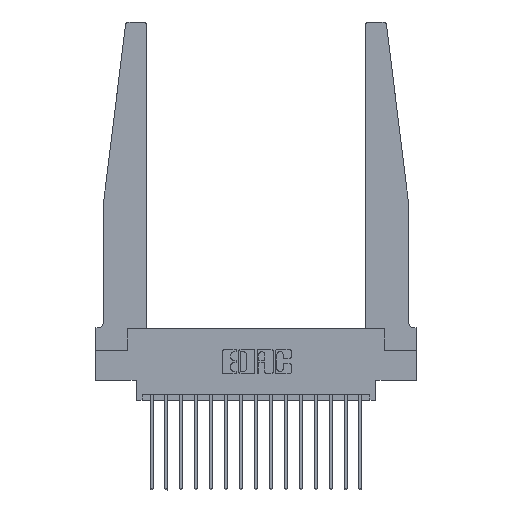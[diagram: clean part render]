
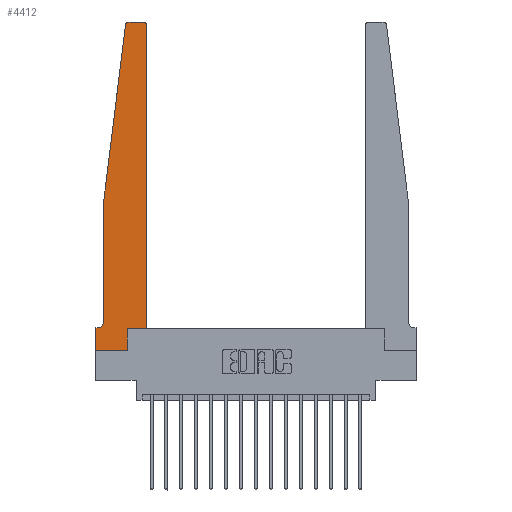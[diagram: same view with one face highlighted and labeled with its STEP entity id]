
A CAD part, top view. The second image highlights one B-rep face of the part: STEP entity #4412.
In plain terms, the highlighted planar face has unit normal (0, 0, 1).
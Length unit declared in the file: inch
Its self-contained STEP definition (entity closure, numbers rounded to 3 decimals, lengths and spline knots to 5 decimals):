
#121 = ORIENTED_EDGE ( 'NONE', *, *, #9849, .T. ) ;
#164 = DIRECTION ( 'NONE',  ( 1., 0., 0. ) ) ;
#223 = LINE ( 'NONE', #15361, #18182 ) ;
#229 = DIRECTION ( 'NONE',  ( 1., 0., 0. ) ) ;
#516 = LINE ( 'NONE', #5419, #961 ) ;
#643 = VECTOR ( 'NONE', #4997, 39.37008 ) ;
#768 = VERTEX_POINT ( 'NONE', #7733 ) ;
#961 = VECTOR ( 'NONE', #12491, 39.37008 ) ;
#1172 = VERTEX_POINT ( 'NONE', #8192 ) ;
#1193 = EDGE_CURVE ( 'NONE', #768, #3084, #7460, .T. ) ;
#1429 = EDGE_CURVE ( 'NONE', #5966, #18178, #14309, .T. ) ;
#2091 = VERTEX_POINT ( 'NONE', #11715 ) ;
#2338 = EDGE_CURVE ( 'NONE', #12616, #2091, #516, .T. ) ;
#2660 = ORIENTED_EDGE ( 'NONE', *, *, #11470, .T. ) ;
#2821 = ORIENTED_EDGE ( 'NONE', *, *, #5171, .T. ) ;
#2945 = PLANE ( 'NONE',  #18149 ) ;
#2963 = CARTESIAN_POINT ( 'NONE',  ( 0., 0., 0.37 ) ) ;
#3084 = VERTEX_POINT ( 'NONE', #2963 ) ;
#3543 = ORIENTED_EDGE ( 'NONE', *, *, #1429, .T. ) ;
#3628 = CARTESIAN_POINT ( 'NONE',  ( 0.425, 0.18, 0.37 ) ) ;
#4214 = EDGE_CURVE ( 'NONE', #9185, #15497, #4988, .T. ) ;
#4399 = AXIS2_PLACEMENT_3D ( 'NONE', #17159, #8705, #164 ) ;
#4412 = ADVANCED_FACE ( 'NONE', ( #16954 ), #2945, .T. ) ;
#4439 = CARTESIAN_POINT ( 'NONE',  ( 0., 0.1875, 0.37 ) ) ;
#4670 = DIRECTION ( 'NONE',  ( 1., 0., 0. ) ) ;
#4988 = LINE ( 'NONE', #9378, #15846 ) ;
#4997 = DIRECTION ( 'NONE',  ( -1., 0., 0. ) ) ;
#5057 = VERTEX_POINT ( 'NONE', #14268 ) ;
#5171 = EDGE_CURVE ( 'NONE', #3084, #9029, #9197, .T. ) ;
#5419 = CARTESIAN_POINT ( 'NONE',  ( 0.065, 1.25, 0.37 ) ) ;
#5646 = EDGE_CURVE ( 'NONE', #15497, #1172, #17139, .T. ) ;
#5870 = DIRECTION ( 'NONE',  ( 1., 0., 0. ) ) ;
#5888 = CARTESIAN_POINT ( 'NONE',  ( 0.425, 0.18, 0.37 ) ) ;
#5966 = VERTEX_POINT ( 'NONE', #6827 ) ;
#6375 = CARTESIAN_POINT ( 'NONE',  ( 0.065, 0.1875, 0.37 ) ) ;
#6827 = CARTESIAN_POINT ( 'NONE',  ( 0.2605, 0.18, 0.37 ) ) ;
#6844 = CARTESIAN_POINT ( 'NONE',  ( 0., 0., 0.37 ) ) ;
#7391 = CARTESIAN_POINT ( 'NONE',  ( 0.065, 1.25, 0.37 ) ) ;
#7449 = ORIENTED_EDGE ( 'NONE', *, *, #2338, .T. ) ;
#7460 = LINE ( 'NONE', #6844, #14083 ) ;
#7733 = CARTESIAN_POINT ( 'NONE',  ( 0., 0.1875, 0.37 ) ) ;
#7759 = DIRECTION ( 'NONE',  ( 0., 0., -1. ) ) ;
#7791 = EDGE_LOOP ( 'NONE', ( #11201, #15063, #15660, #7449, #16136, #2660, #10846, #2821, #9640, #3543, #15742, #121 ) ) ;
#7834 = AXIS2_PLACEMENT_3D ( 'NONE', #16225, #7759, #17645 ) ;
#7994 = DIRECTION ( 'NONE',  ( -1., 0., 0. ) ) ;
#8192 = CARTESIAN_POINT ( 'NONE',  ( 0.24675, 2.72367, 0.37 ) ) ;
#8348 = DIRECTION ( 'NONE',  ( 0., 0., 1. ) ) ;
#8705 = DIRECTION ( 'NONE',  ( 0., 0., 1. ) ) ;
#9029 = VERTEX_POINT ( 'NONE', #11405 ) ;
#9185 = VERTEX_POINT ( 'NONE', #10270 ) ;
#9197 = LINE ( 'NONE', #14562, #12951 ) ;
#9378 = CARTESIAN_POINT ( 'NONE',  ( 0.25, 2.75, 0.37 ) ) ;
#9390 = LINE ( 'NONE', #3628, #16900 ) ;
#9640 = ORIENTED_EDGE ( 'NONE', *, *, #11027, .T. ) ;
#9849 = EDGE_CURVE ( 'NONE', #15060, #9185, #13245, .T. ) ;
#9928 = CARTESIAN_POINT ( 'NONE',  ( 0.065, 1.25, 0.37 ) ) ;
#10068 = LINE ( 'NONE', #7391, #13785 ) ;
#10270 = CARTESIAN_POINT ( 'NONE',  ( 0.395, 2.75, 0.37 ) ) ;
#10390 = CIRCLE ( 'NONE', #7834, 0.05 ) ;
#10846 = ORIENTED_EDGE ( 'NONE', *, *, #1193, .T. ) ;
#11027 = EDGE_CURVE ( 'NONE', #9029, #5966, #223, .T. ) ;
#11198 = DIRECTION ( 'NONE',  ( 0., 1., 0. ) ) ;
#11201 = ORIENTED_EDGE ( 'NONE', *, *, #4214, .T. ) ;
#11405 = CARTESIAN_POINT ( 'NONE',  ( 0.2605, 0., 0.37 ) ) ;
#11470 = EDGE_CURVE ( 'NONE', #5057, #768, #15737, .T. ) ;
#11715 = CARTESIAN_POINT ( 'NONE',  ( 0.065, 0.2375, 0.37 ) ) ;
#12491 = DIRECTION ( 'NONE',  ( 0., -1., 0. ) ) ;
#12616 = VERTEX_POINT ( 'NONE', #9928 ) ;
#12951 = VECTOR ( 'NONE', #4670, 39.37008 ) ;
#13020 = DIRECTION ( 'NONE',  ( -0.122, -0.992, 0. ) ) ;
#13245 = CIRCLE ( 'NONE', #18094, 0.03 ) ;
#13548 = DIRECTION ( 'NONE',  ( 0., 1., 0. ) ) ;
#13785 = VECTOR ( 'NONE', #13020, 39.37008 ) ;
#13861 = DIRECTION ( 'NONE',  ( 0., -1., 0. ) ) ;
#14070 = EDGE_CURVE ( 'NONE', #2091, #5057, #10390, .T. ) ;
#14083 = VECTOR ( 'NONE', #13861, 39.37008 ) ;
#14268 = CARTESIAN_POINT ( 'NONE',  ( 0.015, 0.1875, 0.37 ) ) ;
#14309 = LINE ( 'NONE', #5888, #15180 ) ;
#14352 = DIRECTION ( 'NONE',  ( 0., 0., 1. ) ) ;
#14562 = CARTESIAN_POINT ( 'NONE',  ( 0., 0., 0.37 ) ) ;
#15060 = VERTEX_POINT ( 'NONE', #17776 ) ;
#15063 = ORIENTED_EDGE ( 'NONE', *, *, #5646, .T. ) ;
#15180 = VECTOR ( 'NONE', #229, 39.37008 ) ;
#15361 = CARTESIAN_POINT ( 'NONE',  ( 0.2605, 0.18, 0.37 ) ) ;
#15497 = VERTEX_POINT ( 'NONE', #17451 ) ;
#15660 = ORIENTED_EDGE ( 'NONE', *, *, #17291, .T. ) ;
#15737 = LINE ( 'NONE', #6375, #643 ) ;
#15742 = ORIENTED_EDGE ( 'NONE', *, *, #17556, .T. ) ;
#15772 = CARTESIAN_POINT ( 'NONE',  ( 0.425, 0.18, 0.37 ) ) ;
#15846 = VECTOR ( 'NONE', #7994, 39.37008 ) ;
#16136 = ORIENTED_EDGE ( 'NONE', *, *, #14070, .T. ) ;
#16225 = CARTESIAN_POINT ( 'NONE',  ( 0.015, 0.2375, 0.37 ) ) ;
#16828 = CARTESIAN_POINT ( 'NONE',  ( 0.395, 2.72, 0.37 ) ) ;
#16900 = VECTOR ( 'NONE', #13548, 39.37008 ) ;
#16954 = FACE_OUTER_BOUND ( 'NONE', #7791, .T. ) ;
#17139 = CIRCLE ( 'NONE', #4399, 0.03 ) ;
#17159 = CARTESIAN_POINT ( 'NONE',  ( 0.27653, 2.72, 0.37 ) ) ;
#17291 = EDGE_CURVE ( 'NONE', #1172, #12616, #10068, .T. ) ;
#17451 = CARTESIAN_POINT ( 'NONE',  ( 0.27653, 2.75, 0.37 ) ) ;
#17556 = EDGE_CURVE ( 'NONE', #18178, #15060, #9390, .T. ) ;
#17645 = DIRECTION ( 'NONE',  ( -1., 0., 0. ) ) ;
#17776 = CARTESIAN_POINT ( 'NONE',  ( 0.425, 2.72, 0.37 ) ) ;
#18094 = AXIS2_PLACEMENT_3D ( 'NONE', #16828, #8348, #18235 ) ;
#18149 = AXIS2_PLACEMENT_3D ( 'NONE', #4439, #14352, #5870 ) ;
#18178 = VERTEX_POINT ( 'NONE', #15772 ) ;
#18182 = VECTOR ( 'NONE', #11198, 39.37008 ) ;
#18235 = DIRECTION ( 'NONE',  ( 1., 0., 0. ) ) ;
